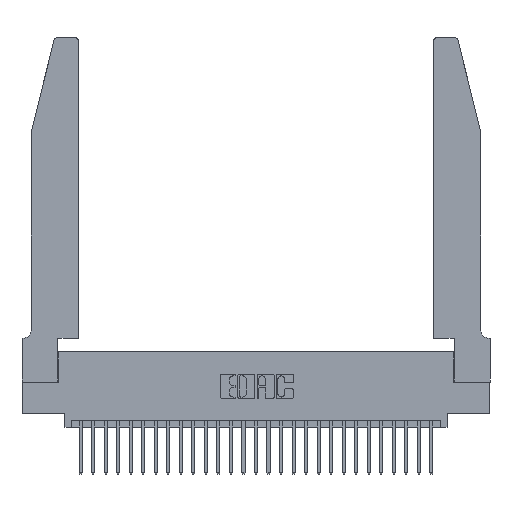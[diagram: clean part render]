
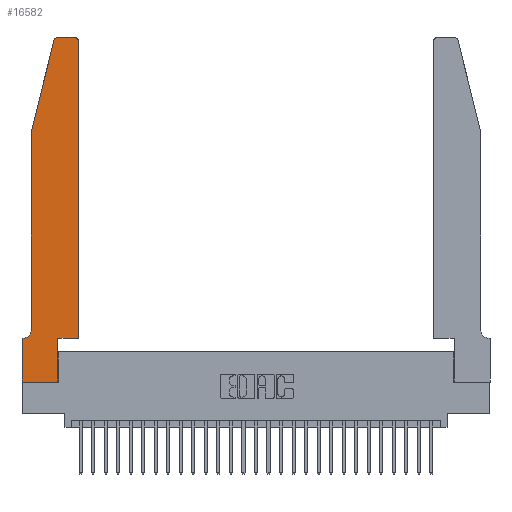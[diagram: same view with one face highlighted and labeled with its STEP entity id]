
A CAD part, top view. The second image highlights one B-rep face of the part: STEP entity #16582.
In plain terms, the highlighted planar face has unit normal (0, 0, 1).
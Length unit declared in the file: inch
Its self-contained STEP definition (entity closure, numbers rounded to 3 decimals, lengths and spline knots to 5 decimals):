
#3 = VECTOR ( 'NONE', #10814, 39.37008 ) ;
#1064 = EDGE_CURVE ( 'NONE', #29357, #2298, #12059, .T. ) ;
#1096 = ORIENTED_EDGE ( 'NONE', *, *, #18779, .T. ) ;
#1173 = CARTESIAN_POINT ( 'NONE',  ( 0.284, 2.75, 0.37 ) ) ;
#1397 = CARTESIAN_POINT ( 'NONE',  ( 0., 0., 0.37 ) ) ;
#1488 = AXIS2_PLACEMENT_3D ( 'NONE', #13785, #2380, #18325 ) ;
#1729 = ORIENTED_EDGE ( 'NONE', *, *, #13316, .T. ) ;
#2014 = DIRECTION ( 'NONE',  ( 0., -1., 0. ) ) ;
#2191 = PLANE ( 'NONE',  #1488 ) ;
#2239 = DIRECTION ( 'NONE',  ( 0., 1., 0. ) ) ;
#2298 = VERTEX_POINT ( 'NONE', #23888 ) ;
#2380 = DIRECTION ( 'NONE',  ( 0., 0., 1. ) ) ;
#2724 = CARTESIAN_POINT ( 'NONE',  ( 0.0755, 2., 0.37 ) ) ;
#3353 = CARTESIAN_POINT ( 'NONE',  ( 0.25487, 2.72718, 0.37 ) ) ;
#3367 = FACE_OUTER_BOUND ( 'NONE', #26128, .T. ) ;
#4328 = CARTESIAN_POINT ( 'NONE',  ( 0.0055, 0.42, 0.37 ) ) ;
#4506 = ORIENTED_EDGE ( 'NONE', *, *, #5341, .T. ) ;
#4575 = LINE ( 'NONE', #27195, #9233 ) ;
#4723 = CARTESIAN_POINT ( 'NONE',  ( 0.2605, 2.75, 0.37 ) ) ;
#5044 = DIRECTION ( 'NONE',  ( -0.239, -0.971, 0. ) ) ;
#5108 = VECTOR ( 'NONE', #15515, 39.37008 ) ;
#5341 = EDGE_CURVE ( 'NONE', #22230, #27278, #27740, .T. ) ;
#5537 = CIRCLE ( 'NONE', #21595, 0.07 ) ;
#6326 = CARTESIAN_POINT ( 'NONE',  ( 0., 0., 0.37 ) ) ;
#6616 = DIRECTION ( 'NONE',  ( -1., 0., 0. ) ) ;
#6785 = VERTEX_POINT ( 'NONE', #17323 ) ;
#6943 = ORIENTED_EDGE ( 'NONE', *, *, #23579, .T. ) ;
#7013 = EDGE_CURVE ( 'NONE', #2298, #29279, #4575, .T. ) ;
#7146 = CIRCLE ( 'NONE', #14841, 0.03 ) ;
#7438 = DIRECTION ( 'NONE',  ( 0., 1., 0. ) ) ;
#7855 = DIRECTION ( 'NONE',  ( 0., 0., 1. ) ) ;
#8560 = CARTESIAN_POINT ( 'NONE',  ( 0., 0., 0.37 ) ) ;
#9008 = CARTESIAN_POINT ( 'NONE',  ( 0.4505, 2.72, 0.37 ) ) ;
#9053 = AXIS2_PLACEMENT_3D ( 'NONE', #21455, #7855, #23724 ) ;
#9233 = VECTOR ( 'NONE', #2239, 39.37008 ) ;
#9350 = EDGE_CURVE ( 'NONE', #18684, #14136, #5537, .T. ) ;
#10531 = VECTOR ( 'NONE', #24351, 39.37008 ) ;
#10814 = DIRECTION ( 'NONE',  ( -1., 0., 0. ) ) ;
#10998 = VERTEX_POINT ( 'NONE', #3353 ) ;
#10999 = DIRECTION ( 'NONE',  ( 0., 0., 1. ) ) ;
#11240 = LINE ( 'NONE', #6326, #5108 ) ;
#11423 = LINE ( 'NONE', #15706, #22730 ) ;
#11950 = LINE ( 'NONE', #12981, #10531 ) ;
#12059 = LINE ( 'NONE', #1397, #23377 ) ;
#12187 = LINE ( 'NONE', #22064, #3 ) ;
#12863 = VERTEX_POINT ( 'NONE', #25928 ) ;
#12981 = CARTESIAN_POINT ( 'NONE',  ( 0.4505, 0.35, 0.37 ) ) ;
#13172 = ORIENTED_EDGE ( 'NONE', *, *, #22374, .T. ) ;
#13316 = EDGE_CURVE ( 'NONE', #20000, #10998, #7146, .T. ) ;
#13780 = CIRCLE ( 'NONE', #9053, 0.03 ) ;
#13785 = CARTESIAN_POINT ( 'NONE',  ( 0., 0.35, 0.37 ) ) ;
#14118 = EDGE_CURVE ( 'NONE', #25157, #18684, #11423, .T. ) ;
#14136 = VERTEX_POINT ( 'NONE', #24796 ) ;
#14609 = ORIENTED_EDGE ( 'NONE', *, *, #14118, .T. ) ;
#14841 = AXIS2_PLACEMENT_3D ( 'NONE', #24535, #10999, #26802 ) ;
#15515 = DIRECTION ( 'NONE',  ( 0., -1., 0. ) ) ;
#15706 = CARTESIAN_POINT ( 'NONE',  ( 0.0755, 2., 0.37 ) ) ;
#15734 = VECTOR ( 'NONE', #7438, 39.37008 ) ;
#16099 = DIRECTION ( 'NONE',  ( -1., 0., 0. ) ) ;
#16498 = ORIENTED_EDGE ( 'NONE', *, *, #9350, .T. ) ;
#16582 = ADVANCED_FACE ( 'NONE', ( #3367 ), #2191, .T. ) ;
#17323 = CARTESIAN_POINT ( 'NONE',  ( 0.4205, 2.75, 0.37 ) ) ;
#17767 = VECTOR ( 'NONE', #5044, 39.37008 ) ;
#18325 = DIRECTION ( 'NONE',  ( 1., 0., 0. ) ) ;
#18684 = VERTEX_POINT ( 'NONE', #23954 ) ;
#18779 = EDGE_CURVE ( 'NONE', #14136, #12863, #12187, .T. ) ;
#18940 = ORIENTED_EDGE ( 'NONE', *, *, #1064, .T. ) ;
#19178 = LINE ( 'NONE', #2724, #17767 ) ;
#19545 = ORIENTED_EDGE ( 'NONE', *, *, #7013, .T. ) ;
#20000 = VERTEX_POINT ( 'NONE', #1173 ) ;
#20236 = DIRECTION ( 'NONE',  ( 0., 0., -1. ) ) ;
#20416 = CARTESIAN_POINT ( 'NONE',  ( 0.4505, 0.35, 0.37 ) ) ;
#21040 = CARTESIAN_POINT ( 'NONE',  ( 0.4505, 0.35, 0.37 ) ) ;
#21100 = EDGE_CURVE ( 'NONE', #10998, #25157, #19178, .T. ) ;
#21455 = CARTESIAN_POINT ( 'NONE',  ( 0.4205, 2.72, 0.37 ) ) ;
#21595 = AXIS2_PLACEMENT_3D ( 'NONE', #4328, #20236, #6616 ) ;
#21687 = EDGE_CURVE ( 'NONE', #6785, #20000, #23038, .T. ) ;
#21710 = DIRECTION ( 'NONE',  ( 1., 0., 0. ) ) ;
#22064 = CARTESIAN_POINT ( 'NONE',  ( 0.0755, 0.35, 0.37 ) ) ;
#22230 = VERTEX_POINT ( 'NONE', #20416 ) ;
#22374 = EDGE_CURVE ( 'NONE', #29279, #22230, #11950, .T. ) ;
#22730 = VECTOR ( 'NONE', #2014, 39.37008 ) ;
#23038 = LINE ( 'NONE', #4723, #26926 ) ;
#23377 = VECTOR ( 'NONE', #21710, 39.37008 ) ;
#23579 = EDGE_CURVE ( 'NONE', #12863, #29357, #11240, .T. ) ;
#23724 = DIRECTION ( 'NONE',  ( 1., 0., 0. ) ) ;
#23888 = CARTESIAN_POINT ( 'NONE',  ( 0.2865, 0., 0.37 ) ) ;
#23954 = CARTESIAN_POINT ( 'NONE',  ( 0.0755, 0.42, 0.37 ) ) ;
#24351 = DIRECTION ( 'NONE',  ( 1., 0., 0. ) ) ;
#24535 = CARTESIAN_POINT ( 'NONE',  ( 0.284, 2.72, 0.37 ) ) ;
#24796 = CARTESIAN_POINT ( 'NONE',  ( 0.0055, 0.35, 0.37 ) ) ;
#24890 = ORIENTED_EDGE ( 'NONE', *, *, #21100, .T. ) ;
#25157 = VERTEX_POINT ( 'NONE', #27658 ) ;
#25459 = ORIENTED_EDGE ( 'NONE', *, *, #21687, .T. ) ;
#25928 = CARTESIAN_POINT ( 'NONE',  ( 0., 0.35, 0.37 ) ) ;
#26128 = EDGE_LOOP ( 'NONE', ( #25459, #1729, #24890, #14609, #16498, #1096, #6943, #18940, #19545, #13172, #4506, #28586 ) ) ;
#26392 = CARTESIAN_POINT ( 'NONE',  ( 0.2865, 0.35, 0.37 ) ) ;
#26802 = DIRECTION ( 'NONE',  ( 1., 0., 0. ) ) ;
#26926 = VECTOR ( 'NONE', #16099, 39.37008 ) ;
#27195 = CARTESIAN_POINT ( 'NONE',  ( 0.2865, 0.35, 0.37 ) ) ;
#27278 = VERTEX_POINT ( 'NONE', #9008 ) ;
#27658 = CARTESIAN_POINT ( 'NONE',  ( 0.0755, 2., 0.37 ) ) ;
#27740 = LINE ( 'NONE', #21040, #15734 ) ;
#28586 = ORIENTED_EDGE ( 'NONE', *, *, #29114, .T. ) ;
#29114 = EDGE_CURVE ( 'NONE', #27278, #6785, #13780, .T. ) ;
#29279 = VERTEX_POINT ( 'NONE', #26392 ) ;
#29357 = VERTEX_POINT ( 'NONE', #8560 ) ;
